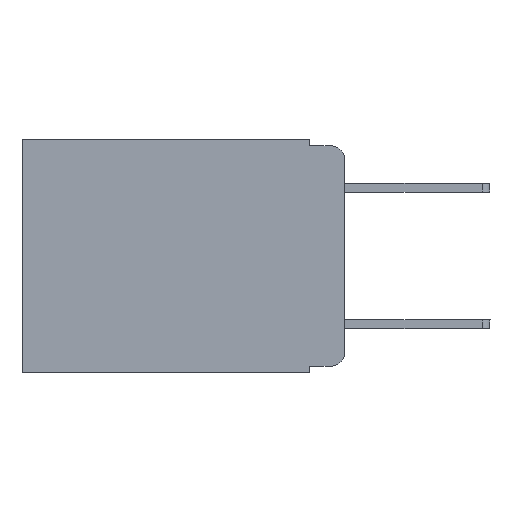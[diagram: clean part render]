
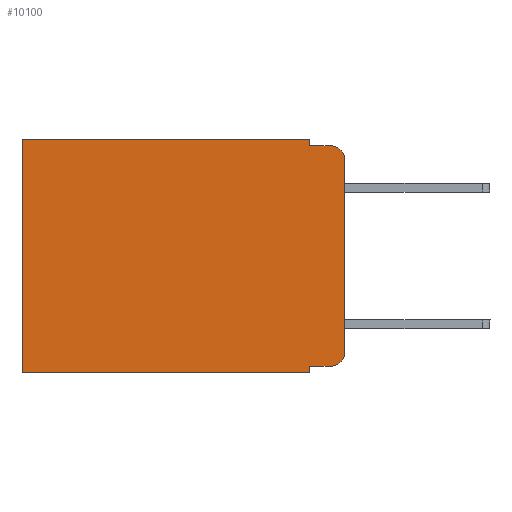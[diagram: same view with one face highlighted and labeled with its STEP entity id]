
A CAD part, left-side view. The second image highlights one B-rep face of the part: STEP entity #10100.
In plain terms, the highlighted planar face has unit normal (-1, 0, 0).
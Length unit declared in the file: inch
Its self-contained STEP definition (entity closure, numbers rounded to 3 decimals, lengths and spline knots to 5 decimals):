
#34 = ORIENTED_EDGE ( 'NONE', *, *, #15218, .F. ) ;
#188 = VECTOR ( 'NONE', #12648, 39.37008 ) ;
#289 = ORIENTED_EDGE ( 'NONE', *, *, #5444, .F. ) ;
#1096 = LINE ( 'NONE', #5392, #1701 ) ;
#1388 = CIRCLE ( 'NONE', #10466, 0.02 ) ;
#1593 = CARTESIAN_POINT ( 'NONE',  ( 0.298, 0.473, 0. ) ) ;
#1683 = CARTESIAN_POINT ( 'NONE',  ( 0.298, 0.051, -0.01 ) ) ;
#1701 = VECTOR ( 'NONE', #12057, 39.37008 ) ;
#1856 = CARTESIAN_POINT ( 'NONE',  ( 0.298, 0., -0.343 ) ) ;
#1923 = FACE_OUTER_BOUND ( 'NONE', #14040, .T. ) ;
#1926 = LINE ( 'NONE', #1856, #15568 ) ;
#1988 = ORIENTED_EDGE ( 'NONE', *, *, #10094, .T. ) ;
#2183 = CARTESIAN_POINT ( 'NONE',  ( 0.298, 0.051, 0. ) ) ;
#2495 = ORIENTED_EDGE ( 'NONE', *, *, #5018, .T. ) ;
#2587 = CARTESIAN_POINT ( 'NONE',  ( 0.298, 0.051, 0. ) ) ;
#2945 = CARTESIAN_POINT ( 'NONE',  ( 0.298, 0.051, -0.333 ) ) ;
#3000 = VECTOR ( 'NONE', #5238, 39.37008 ) ;
#3381 = CARTESIAN_POINT ( 'NONE',  ( 0.298, 0., 0. ) ) ;
#3468 = VERTEX_POINT ( 'NONE', #12085 ) ;
#4122 = AXIS2_PLACEMENT_3D ( 'NONE', #10406, #6556, #17125 ) ;
#4306 = VERTEX_POINT ( 'NONE', #5748 ) ;
#4307 = DIRECTION ( 'NONE',  ( 0., 1., 0. ) ) ;
#4362 = VERTEX_POINT ( 'NONE', #15014 ) ;
#4827 = LINE ( 'NONE', #15778, #3000 ) ;
#4875 = LINE ( 'NONE', #5303, #15031 ) ;
#5018 = EDGE_CURVE ( 'NONE', #4362, #11426, #5085, .T. ) ;
#5085 = CIRCLE ( 'NONE', #4122, 0.02 ) ;
#5238 = DIRECTION ( 'NONE',  ( 0., -1., 0. ) ) ;
#5284 = CARTESIAN_POINT ( 'NONE',  ( 0.298, 0., 0. ) ) ;
#5303 = CARTESIAN_POINT ( 'NONE',  ( 0.298, 0., 0. ) ) ;
#5392 = CARTESIAN_POINT ( 'NONE',  ( 0.298, 0.473, 0. ) ) ;
#5444 = EDGE_CURVE ( 'NONE', #11329, #8180, #11716, .T. ) ;
#5448 = DIRECTION ( 'NONE',  ( 0., 0., -1. ) ) ;
#5505 = DIRECTION ( 'NONE',  ( -1., 0., 0. ) ) ;
#5748 = CARTESIAN_POINT ( 'NONE',  ( 0.298, 0.051, -0.343 ) ) ;
#5975 = EDGE_CURVE ( 'NONE', #8180, #3468, #4827, .T. ) ;
#6461 = CARTESIAN_POINT ( 'NONE',  ( 0.298, 0.473, -0.343 ) ) ;
#6480 = DIRECTION ( 'NONE',  ( 0., 0., -1. ) ) ;
#6556 = DIRECTION ( 'NONE',  ( -1., 0., 0. ) ) ;
#6799 = CARTESIAN_POINT ( 'NONE',  ( 0.298, 0.051, 0. ) ) ;
#7003 = ORIENTED_EDGE ( 'NONE', *, *, #16869, .T. ) ;
#7217 = EDGE_CURVE ( 'NONE', #4306, #12447, #1926, .T. ) ;
#7263 = DIRECTION ( 'NONE',  ( 0., 1., 0. ) ) ;
#7623 = LINE ( 'NONE', #9975, #188 ) ;
#7785 = VECTOR ( 'NONE', #8685, 39.37008 ) ;
#8027 = CARTESIAN_POINT ( 'NONE',  ( 0.298, 0.02, -0.03 ) ) ;
#8136 = DIRECTION ( 'NONE',  ( 1., 0., 0. ) ) ;
#8180 = VERTEX_POINT ( 'NONE', #1683 ) ;
#8685 = DIRECTION ( 'NONE',  ( 0., 0., -1. ) ) ;
#8888 = CARTESIAN_POINT ( 'NONE',  ( 0.298, 0., -0.313 ) ) ;
#9186 = ORIENTED_EDGE ( 'NONE', *, *, #7217, .F. ) ;
#9671 = LINE ( 'NONE', #3381, #14054 ) ;
#9975 = CARTESIAN_POINT ( 'NONE',  ( 0.298, 0.051, -0.333 ) ) ;
#10013 = VERTEX_POINT ( 'NONE', #12833 ) ;
#10094 = EDGE_CURVE ( 'NONE', #11280, #12447, #1096, .T. ) ;
#10100 = ADVANCED_FACE ( 'NONE', ( #1923 ), #10714, .F. ) ;
#10406 = CARTESIAN_POINT ( 'NONE',  ( 0.298, 0.02, -0.313 ) ) ;
#10466 = AXIS2_PLACEMENT_3D ( 'NONE', #8027, #5505, #5448 ) ;
#10714 = PLANE ( 'NONE',  #11840 ) ;
#10749 = DIRECTION ( 'NONE',  ( 0., 0., -1. ) ) ;
#10920 = LINE ( 'NONE', #2183, #7785 ) ;
#11280 = VERTEX_POINT ( 'NONE', #1593 ) ;
#11329 = VERTEX_POINT ( 'NONE', #6799 ) ;
#11426 = VERTEX_POINT ( 'NONE', #8888 ) ;
#11716 = LINE ( 'NONE', #2587, #15631 ) ;
#11840 = AXIS2_PLACEMENT_3D ( 'NONE', #5284, #8136, #13288 ) ;
#11853 = VERTEX_POINT ( 'NONE', #2945 ) ;
#12057 = DIRECTION ( 'NONE',  ( 0., 0., -1. ) ) ;
#12085 = CARTESIAN_POINT ( 'NONE',  ( 0.298, 0.02, -0.01 ) ) ;
#12447 = VERTEX_POINT ( 'NONE', #6461 ) ;
#12648 = DIRECTION ( 'NONE',  ( 0., -1., 0. ) ) ;
#12833 = CARTESIAN_POINT ( 'NONE',  ( 0.298, 0., -0.03 ) ) ;
#13288 = DIRECTION ( 'NONE',  ( 0., 0., -1. ) ) ;
#14040 = EDGE_LOOP ( 'NONE', ( #15684, #7003, #15421, #289, #15122, #1988, #9186, #34, #14454, #2495 ) ) ;
#14054 = VECTOR ( 'NONE', #7263, 39.37008 ) ;
#14082 = EDGE_CURVE ( 'NONE', #11329, #11280, #9671, .T. ) ;
#14454 = ORIENTED_EDGE ( 'NONE', *, *, #15194, .T. ) ;
#15014 = CARTESIAN_POINT ( 'NONE',  ( 0.298, 0.02, -0.333 ) ) ;
#15031 = VECTOR ( 'NONE', #10749, 39.37008 ) ;
#15122 = ORIENTED_EDGE ( 'NONE', *, *, #14082, .T. ) ;
#15194 = EDGE_CURVE ( 'NONE', #11853, #4362, #7623, .T. ) ;
#15218 = EDGE_CURVE ( 'NONE', #11853, #4306, #10920, .T. ) ;
#15421 = ORIENTED_EDGE ( 'NONE', *, *, #5975, .F. ) ;
#15568 = VECTOR ( 'NONE', #4307, 39.37008 ) ;
#15631 = VECTOR ( 'NONE', #6480, 39.37008 ) ;
#15684 = ORIENTED_EDGE ( 'NONE', *, *, #16143, .F. ) ;
#15778 = CARTESIAN_POINT ( 'NONE',  ( 0.298, 0.051, -0.01 ) ) ;
#16143 = EDGE_CURVE ( 'NONE', #10013, #11426, #4875, .T. ) ;
#16869 = EDGE_CURVE ( 'NONE', #10013, #3468, #1388, .T. ) ;
#17125 = DIRECTION ( 'NONE',  ( 0., 0., -1. ) ) ;
